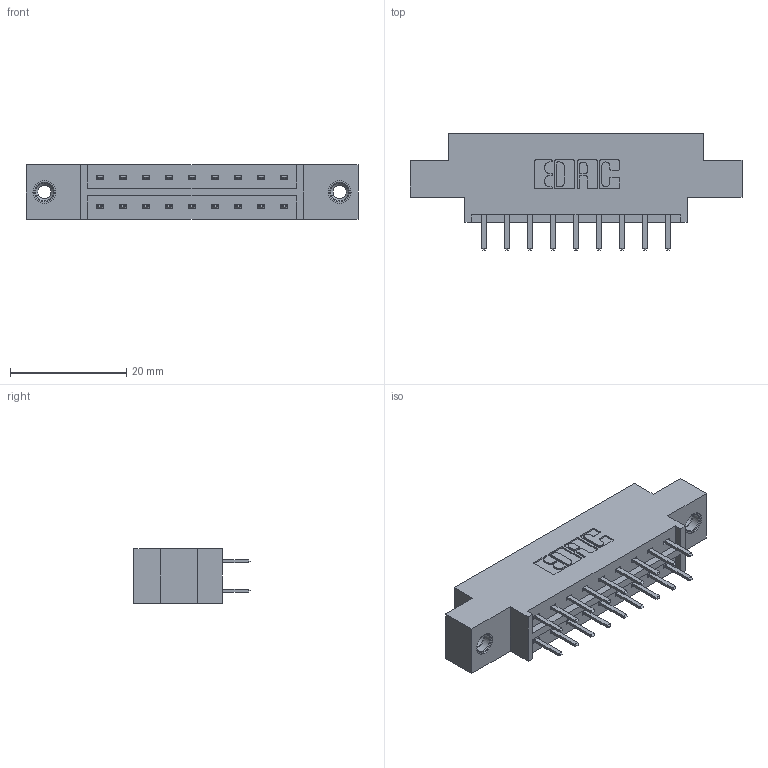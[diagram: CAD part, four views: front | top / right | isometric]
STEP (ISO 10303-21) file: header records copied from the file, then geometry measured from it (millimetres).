
FILE_DESCRIPTION (( 'STEP AP203' ), '1' );
FILE_NAME ('833-018-520-808.STEP', '2020-05-31T21:10:28', ( '' ), ( '' ), 'SwSTEP 2.0', 'SolidWorks 2020', '' );
FILE_SCHEMA (( 'CONFIG_CONTROL_DESIGN' ));
Length unit declared in the file: inch
Products named in the file (4): 833 Part_Offset - .156 Dia - TI; 345-250-001_345-250-003-102; 833-018-520-808; 345-292-001_345-293-120
Assembly tree (21 placements, depth 2):
  833-018-520-808
    833 Part_Offset - .156 Dia - TI
    345-292-001_345-293-120  x18
    345-250-001_345-250-003-102  x2
Bounding box: 57.2 x 20.02 x 9.4 mm (x, y, z)
Volume: 5289 mm3; surface area: 6120 mm2
Topology: 21 solids, 21 shells, 1186 faces, 3393 edges, 2206 vertices
Faces by surface type: plane 790, cylinder 380, cone 12, torus 4
Entity records: 11490 total; most frequent: CARTESIAN_POINT 1941, ORIENTED_EDGE 1858, DIRECTION 1735, EDGE_CURVE 929, LINE 777, VECTOR 777, VERTEX_POINT 612, AXIS2_PLACEMENT_3D 479
